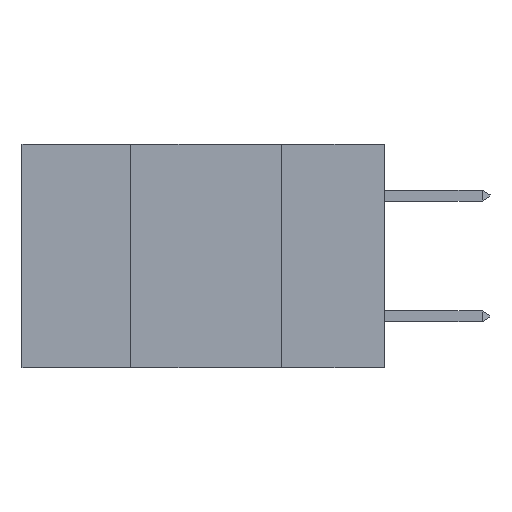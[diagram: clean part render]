
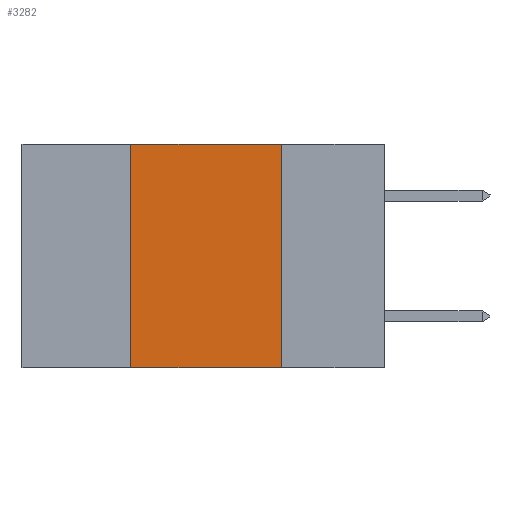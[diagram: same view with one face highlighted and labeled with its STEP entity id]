
A CAD part, left-side view. The second image highlights one B-rep face of the part: STEP entity #3282.
In plain terms, the highlighted planar face has unit normal (-1, 0, 0).
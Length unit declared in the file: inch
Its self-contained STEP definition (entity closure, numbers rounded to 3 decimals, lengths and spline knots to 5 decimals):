
#36 = DIRECTION ( 'NONE',  ( 0., -1., 0. ) ) ;
#347 = PLANE ( 'NONE',  #6016 ) ;
#433 = DIRECTION ( 'NONE',  ( 0., 0., -1. ) ) ;
#1059 = ORIENTED_EDGE ( 'NONE', *, *, #7818, .F. ) ;
#1087 = LINE ( 'NONE', #6203, #6753 ) ;
#1711 = ORIENTED_EDGE ( 'NONE', *, *, #2232, .F. ) ;
#2174 = VERTEX_POINT ( 'NONE', #4335 ) ;
#2232 = EDGE_CURVE ( 'NONE', #2174, #12439, #3917, .T. ) ;
#2963 = EDGE_LOOP ( 'NONE', ( #1711, #1059, #4135, #11809 ) ) ;
#3276 = CARTESIAN_POINT ( 'NONE',  ( 0., 0.42, 0. ) ) ;
#3282 = ADVANCED_FACE ( 'NONE', ( #7806 ), #347, .F. ) ;
#3917 = LINE ( 'NONE', #10610, #10052 ) ;
#4135 = ORIENTED_EDGE ( 'NONE', *, *, #10363, .F. ) ;
#4211 = VERTEX_POINT ( 'NONE', #6977 ) ;
#4335 = CARTESIAN_POINT ( 'NONE',  ( 0., 0.17, 0. ) ) ;
#4370 = VECTOR ( 'NONE', #36, 39.37008 ) ;
#4468 = CARTESIAN_POINT ( 'NONE',  ( 0., 0.6, 0. ) ) ;
#4920 = VECTOR ( 'NONE', #8400, 39.37008 ) ;
#5263 = DIRECTION ( 'NONE',  ( 0., -1., 0. ) ) ;
#6016 = AXIS2_PLACEMENT_3D ( 'NONE', #4468, #11482, #433 ) ;
#6203 = CARTESIAN_POINT ( 'NONE',  ( 0., 0.6, -0.37 ) ) ;
#6753 = VECTOR ( 'NONE', #5263, 39.37008 ) ;
#6977 = CARTESIAN_POINT ( 'NONE',  ( 0., 0.42, 0. ) ) ;
#7342 = CARTESIAN_POINT ( 'NONE',  ( 0., 0.17, -0.37 ) ) ;
#7806 = FACE_OUTER_BOUND ( 'NONE', #2963, .T. ) ;
#7818 = EDGE_CURVE ( 'NONE', #4211, #2174, #12685, .T. ) ;
#8400 = DIRECTION ( 'NONE',  ( 0., 0., 1. ) ) ;
#8767 = DIRECTION ( 'NONE',  ( 0., 0., -1. ) ) ;
#9494 = CARTESIAN_POINT ( 'NONE',  ( 0., 0.42, -0.37 ) ) ;
#10052 = VECTOR ( 'NONE', #8767, 39.37008 ) ;
#10363 = EDGE_CURVE ( 'NONE', #12110, #4211, #12158, .T. ) ;
#10610 = CARTESIAN_POINT ( 'NONE',  ( 0., 0.17, 0. ) ) ;
#11063 = CARTESIAN_POINT ( 'NONE',  ( 0., 0.6, 0. ) ) ;
#11482 = DIRECTION ( 'NONE',  ( 1., 0., 0. ) ) ;
#11809 = ORIENTED_EDGE ( 'NONE', *, *, #12547, .T. ) ;
#12110 = VERTEX_POINT ( 'NONE', #9494 ) ;
#12158 = LINE ( 'NONE', #3276, #4920 ) ;
#12439 = VERTEX_POINT ( 'NONE', #7342 ) ;
#12547 = EDGE_CURVE ( 'NONE', #12110, #12439, #1087, .T. ) ;
#12685 = LINE ( 'NONE', #11063, #4370 ) ;
